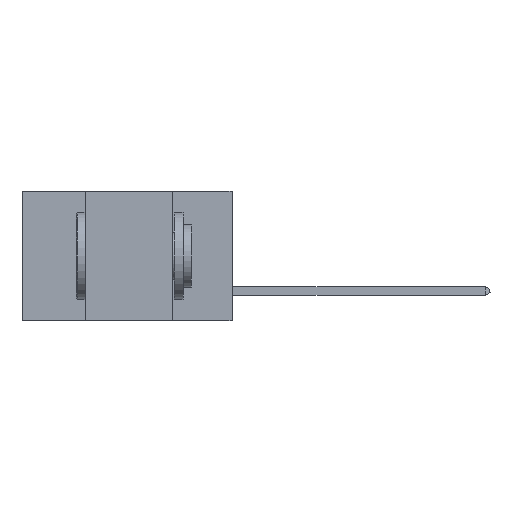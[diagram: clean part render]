
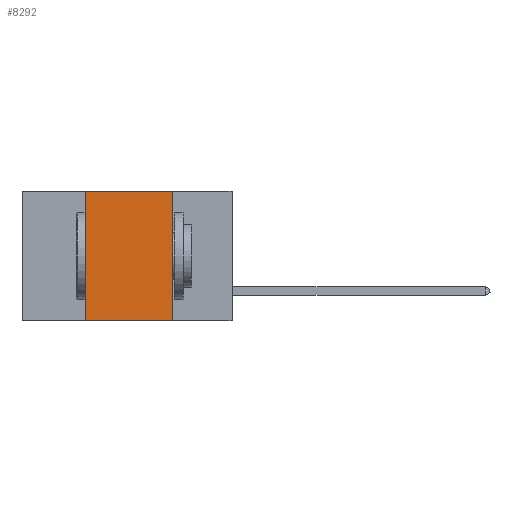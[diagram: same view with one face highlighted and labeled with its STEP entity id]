
A CAD part, left-side view. The second image highlights one B-rep face of the part: STEP entity #8292.
In plain terms, the highlighted planar face has unit normal (-1, 0, 0).
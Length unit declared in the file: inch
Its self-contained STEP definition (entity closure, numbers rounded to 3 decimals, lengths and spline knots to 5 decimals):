
#5 = CARTESIAN_POINT ( 'NONE',  ( 0., 0.6, 0. ) ) ;
#320 = DIRECTION ( 'NONE',  ( 0., 0., -1. ) ) ;
#379 = CARTESIAN_POINT ( 'NONE',  ( 0., 0.6, -0.37 ) ) ;
#463 = CARTESIAN_POINT ( 'NONE',  ( 0., 0.17, 0. ) ) ;
#1797 = DIRECTION ( 'NONE',  ( 0., -1., 0. ) ) ;
#2029 = LINE ( 'NONE', #379, #15457 ) ;
#2412 = CARTESIAN_POINT ( 'NONE',  ( 0., 0.17, -0.37 ) ) ;
#2492 = VECTOR ( 'NONE', #1797, 39.37008 ) ;
#2952 = PLANE ( 'NONE',  #11503 ) ;
#3468 = VERTEX_POINT ( 'NONE', #3722 ) ;
#3535 = CARTESIAN_POINT ( 'NONE',  ( 0., 0.6, 0. ) ) ;
#3557 = LINE ( 'NONE', #5, #2492 ) ;
#3722 = CARTESIAN_POINT ( 'NONE',  ( 0., 0.42, 0. ) ) ;
#3785 = ORIENTED_EDGE ( 'NONE', *, *, #21178, .F. ) ;
#4743 = VECTOR ( 'NONE', #320, 39.37008 ) ;
#4998 = DIRECTION ( 'NONE',  ( 0., 0., 1. ) ) ;
#7048 = EDGE_CURVE ( 'NONE', #3468, #16367, #3557, .T. ) ;
#7477 = CARTESIAN_POINT ( 'NONE',  ( 0., 0.42, -0.37 ) ) ;
#8292 = ADVANCED_FACE ( 'NONE', ( #16120 ), #2952, .F. ) ;
#8592 = ORIENTED_EDGE ( 'NONE', *, *, #14937, .T. ) ;
#10320 = EDGE_LOOP ( 'NONE', ( #13759, #13176, #3785, #8592 ) ) ;
#11503 = AXIS2_PLACEMENT_3D ( 'NONE', #3535, #13738, #17719 ) ;
#13176 = ORIENTED_EDGE ( 'NONE', *, *, #7048, .F. ) ;
#13738 = DIRECTION ( 'NONE',  ( 1., 0., 0. ) ) ;
#13759 = ORIENTED_EDGE ( 'NONE', *, *, #21281, .F. ) ;
#14937 = EDGE_CURVE ( 'NONE', #17081, #16386, #2029, .T. ) ;
#15060 = CARTESIAN_POINT ( 'NONE',  ( 0., 0.42, 0. ) ) ;
#15457 = VECTOR ( 'NONE', #17342, 39.37008 ) ;
#15960 = CARTESIAN_POINT ( 'NONE',  ( 0., 0.17, 0. ) ) ;
#16120 = FACE_OUTER_BOUND ( 'NONE', #10320, .T. ) ;
#16367 = VERTEX_POINT ( 'NONE', #15960 ) ;
#16386 = VERTEX_POINT ( 'NONE', #2412 ) ;
#16547 = LINE ( 'NONE', #463, #4743 ) ;
#17081 = VERTEX_POINT ( 'NONE', #7477 ) ;
#17342 = DIRECTION ( 'NONE',  ( 0., -1., 0. ) ) ;
#17719 = DIRECTION ( 'NONE',  ( 0., 0., -1. ) ) ;
#18408 = VECTOR ( 'NONE', #4998, 39.37008 ) ;
#18972 = LINE ( 'NONE', #15060, #18408 ) ;
#21178 = EDGE_CURVE ( 'NONE', #17081, #3468, #18972, .T. ) ;
#21281 = EDGE_CURVE ( 'NONE', #16367, #16386, #16547, .T. ) ;
